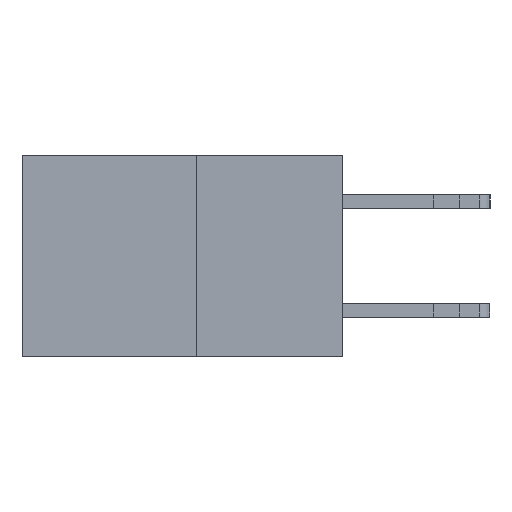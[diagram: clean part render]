
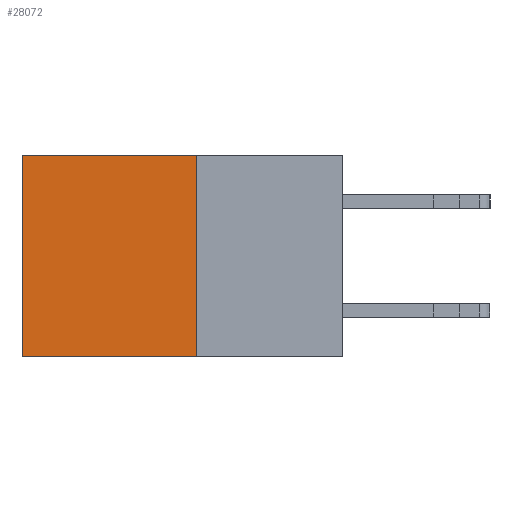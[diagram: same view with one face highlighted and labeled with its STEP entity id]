
A CAD part, left-side view. The second image highlights one B-rep face of the part: STEP entity #28072.
In plain terms, the highlighted planar face has unit normal (-1, 0, 0).
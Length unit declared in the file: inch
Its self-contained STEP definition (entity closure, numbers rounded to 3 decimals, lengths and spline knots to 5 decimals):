
#87 = CARTESIAN_POINT ( 'NONE',  ( 0.277, 0.27, 0. ) ) ;
#418 = DIRECTION ( 'NONE',  ( 0., 1., 0. ) ) ;
#708 = VECTOR ( 'NONE', #15480, 39.37008 ) ;
#1541 = EDGE_CURVE ( 'NONE', #28305, #15733, #13648, .T. ) ;
#1668 = VECTOR ( 'NONE', #17489, 39.37008 ) ;
#3766 = AXIS2_PLACEMENT_3D ( 'NONE', #27697, #13535, #29966 ) ;
#3850 = PLANE ( 'NONE',  #3766 ) ;
#4767 = FACE_OUTER_BOUND ( 'NONE', #23183, .T. ) ;
#4772 = EDGE_CURVE ( 'NONE', #28305, #16275, #29110, .T. ) ;
#5964 = CARTESIAN_POINT ( 'NONE',  ( 0.277, 0.27, -0.37 ) ) ;
#6170 = DIRECTION ( 'NONE',  ( 0., 1., 0. ) ) ;
#6974 = CARTESIAN_POINT ( 'NONE',  ( 0.277, 0.27, -0.37 ) ) ;
#7378 = EDGE_CURVE ( 'NONE', #15733, #24253, #9341, .T. ) ;
#8053 = CARTESIAN_POINT ( 'NONE',  ( 0.277, 0.27, 0. ) ) ;
#8835 = EDGE_CURVE ( 'NONE', #16275, #24253, #19081, .T. ) ;
#9341 = LINE ( 'NONE', #5964, #21396 ) ;
#11855 = CARTESIAN_POINT ( 'NONE',  ( 0.277, 0.59, -0.37 ) ) ;
#13535 = DIRECTION ( 'NONE',  ( 1., 0., 0. ) ) ;
#13648 = LINE ( 'NONE', #6974, #1668 ) ;
#15480 = DIRECTION ( 'NONE',  ( 0., 0., -1. ) ) ;
#15733 = VERTEX_POINT ( 'NONE', #19423 ) ;
#15897 = VECTOR ( 'NONE', #418, 39.37008 ) ;
#16275 = VERTEX_POINT ( 'NONE', #21685 ) ;
#17489 = DIRECTION ( 'NONE',  ( 0., 0., -1. ) ) ;
#19081 = LINE ( 'NONE', #29508, #708 ) ;
#19423 = CARTESIAN_POINT ( 'NONE',  ( 0.277, 0.27, -0.37 ) ) ;
#21396 = VECTOR ( 'NONE', #6170, 39.37008 ) ;
#21685 = CARTESIAN_POINT ( 'NONE',  ( 0.277, 0.59, 0. ) ) ;
#23183 = EDGE_LOOP ( 'NONE', ( #29418, #26150, #26396, #24968 ) ) ;
#24253 = VERTEX_POINT ( 'NONE', #11855 ) ;
#24968 = ORIENTED_EDGE ( 'NONE', *, *, #4772, .T. ) ;
#26150 = ORIENTED_EDGE ( 'NONE', *, *, #7378, .F. ) ;
#26396 = ORIENTED_EDGE ( 'NONE', *, *, #1541, .F. ) ;
#27697 = CARTESIAN_POINT ( 'NONE',  ( 0.277, 0.27, -0.37 ) ) ;
#28072 = ADVANCED_FACE ( 'NONE', ( #4767 ), #3850, .F. ) ;
#28305 = VERTEX_POINT ( 'NONE', #87 ) ;
#29110 = LINE ( 'NONE', #8053, #15897 ) ;
#29418 = ORIENTED_EDGE ( 'NONE', *, *, #8835, .T. ) ;
#29508 = CARTESIAN_POINT ( 'NONE',  ( 0.277, 0.59, -0.37 ) ) ;
#29966 = DIRECTION ( 'NONE',  ( 0., 0., -1. ) ) ;
